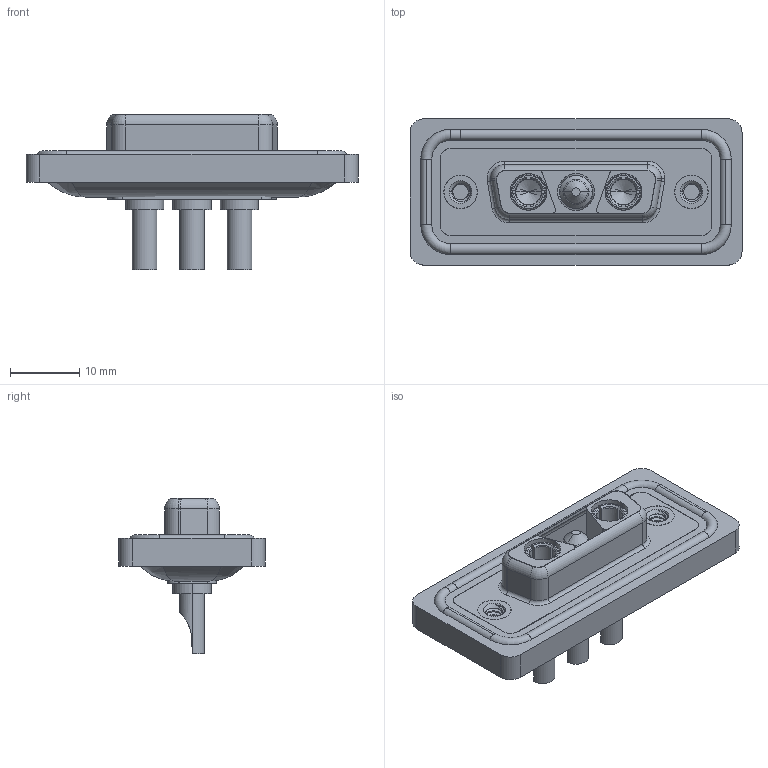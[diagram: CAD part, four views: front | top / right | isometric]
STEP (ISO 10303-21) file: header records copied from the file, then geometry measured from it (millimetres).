
FILE_DESCRIPTION (( 'STEP AP203' ), '1' );
FILE_NAME ('628W3WK3322-2N2.STEP', '2024-04-09T14:37:39', ( '' ), ( '' ), 'SwSTEP 2.0', 'SolidWorks 2023', '' );
FILE_SCHEMA (( 'CONFIG_CONTROL_DESIGN' ));
Length unit declared in the file: millimetre
Products named in the file (8): 628W3WK3322-2N2; 628Combo Shell Front_15 Contacts; 628Combo Housing_3WK3; 628Combo Shell Rear_15 Contacts; Power Pin_20A SC; 628Combo Threaded Rivet_2; Power Socket_20A SC; 628Combo Waterproof Housing_15 Contacts
Assembly tree (9 placements, depth 2):
  628W3WK3322-2N2
    628Combo Housing_3WK3
    628Combo Waterproof Housing_15 Contacts
    628Combo Shell Front_15 Contacts
    628Combo Shell Rear_15 Contacts
    628Combo Threaded Rivet_2  x2
    Power Socket_20A SC  x2
    Power Pin_20A SC
Bounding box: 47.9 x 21.1 x 22.45 mm (x, y, z)
Volume: 5916.5 mm3; surface area: 9752.1 mm2
Topology: 13 solids, 13 shells, 602 faces, 1512 edges, 949 vertices
Faces by surface type: cylinder 267, plane 187, torus 81, cone 53, bspline 14
Entity records: 17645 total; most frequent: CARTESIAN_POINT 4895, DIRECTION 2604, ORIENTED_EDGE 2432, EDGE_CURVE 1216, AXIS2_PLACEMENT_3D 1037, VERTEX_POINT 769, EDGE_LOOP 543, CIRCLE 541
